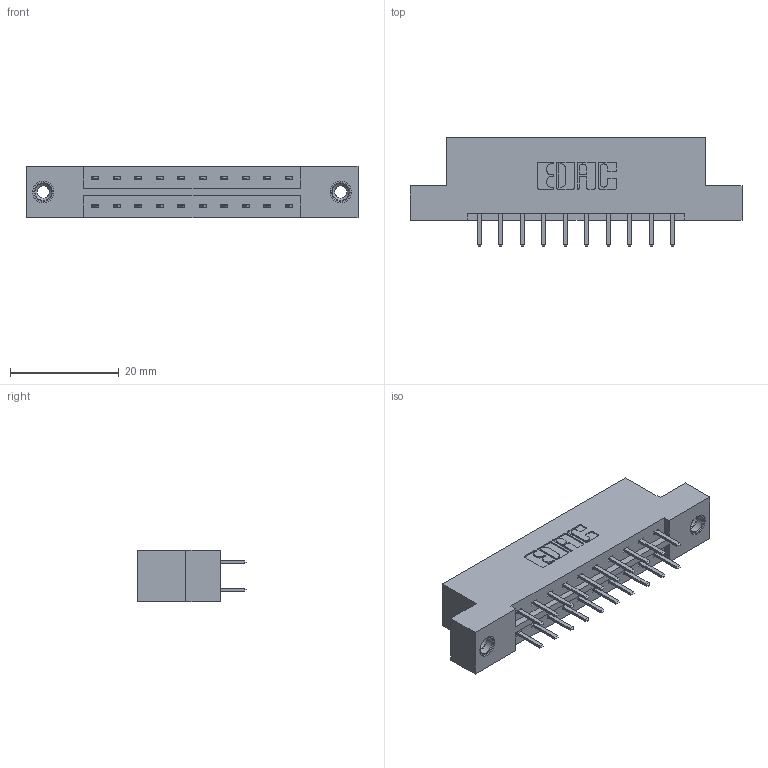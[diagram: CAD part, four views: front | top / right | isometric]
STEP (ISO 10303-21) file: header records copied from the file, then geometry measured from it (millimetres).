
FILE_DESCRIPTION (( 'STEP AP203' ), '1' );
FILE_NAME ('333-020-520-208.STEP', '2018-08-01T23:37:40', ( '' ), ( '' ), 'SwSTEP 2.0', 'SolidWorks 2016', '' );
FILE_SCHEMA (( 'CONFIG_CONTROL_DESIGN' ));
Length unit declared in the file: inch
Products named in the file (4): 333-020-520-208; 333 Part_Flush - .156 Dia - TI; 345-292-001_345-293-120; 345-250-001_345-250-003-102
Assembly tree (23 placements, depth 2):
  333-020-520-208
    333 Part_Flush - .156 Dia - TI
    345-292-001_345-293-120  x20
    345-250-001_345-250-003-102  x2
Bounding box: 61.16 x 20.02 x 9.4 mm (x, y, z)
Volume: 5929.8 mm3; surface area: 6665.2 mm2
Topology: 23 solids, 23 shells, 1294 faces, 3707 edges, 2410 vertices
Faces by surface type: plane 862, cylinder 416, cone 12, torus 4
Entity records: 11872 total; most frequent: CARTESIAN_POINT 2001, ORIENTED_EDGE 1918, DIRECTION 1785, EDGE_CURVE 959, VECTOR 807, LINE 807, VERTEX_POINT 632, AXIS2_PLACEMENT_3D 489
